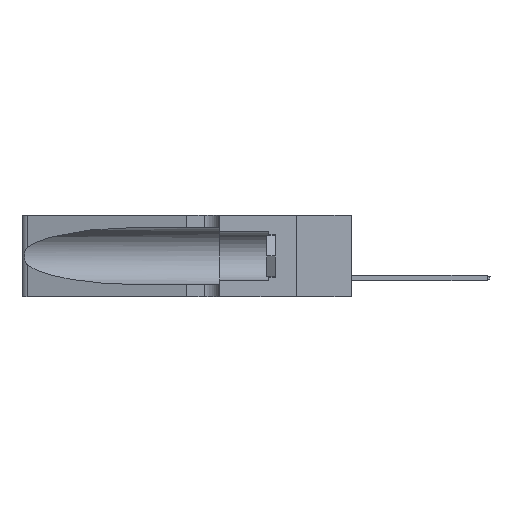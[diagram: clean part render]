
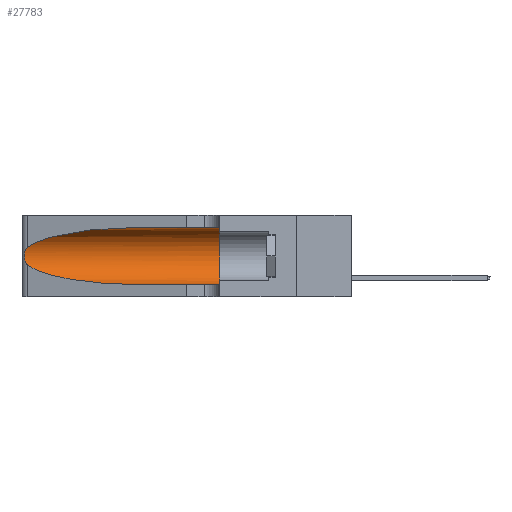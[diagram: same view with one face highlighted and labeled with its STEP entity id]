
A CAD part, left-side view. The second image highlights one B-rep face of the part: STEP entity #27783.
In plain terms, the highlighted cylindrical face has radius 3.308 mm (diameter 6.617 mm), a partial arc.
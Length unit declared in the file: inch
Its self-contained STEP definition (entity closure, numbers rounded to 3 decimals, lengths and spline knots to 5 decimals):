
#856 = DIRECTION ( 'NONE',  ( 0., 0., 1. ) ) ;
#1046 = ORIENTED_EDGE ( 'NONE', *, *, #34919, .F. ) ;
#1336 = CARTESIAN_POINT ( 'NONE',  ( 0.1305, 1.61858, 0.185 ) ) ;
#1360 = CARTESIAN_POINT ( 'NONE',  ( 0.25487, 1.22718, 0.14631 ) ) ;
#1469 = VECTOR ( 'NONE', #13040, 39.37008 ) ;
#3757 = EDGE_CURVE ( 'NONE', #30248, #12861, #10964, .T. ) ;
#3941 = CARTESIAN_POINT ( 'NONE',  ( 0.26017, 1.23833, 0.17102 ) ) ;
#5793 = VERTEX_POINT ( 'NONE', #15947 ) ;
#5950 = VERTEX_POINT ( 'NONE', #10059 ) ;
#6011 = AXIS2_PLACEMENT_3D ( 'NONE', #1336, #27220, #30047 ) ;
#6213 = CYLINDRICAL_SURFACE ( 'NONE', #6011, 0.13025 ) ;
#6783 = VECTOR ( 'NONE', #34614, 39.37008 ) ;
#7017 = EDGE_CURVE ( 'NONE', #27018, #30248, #33963, .T. ) ;
#7101 =( BOUNDED_CURVE ( )  B_SPLINE_CURVE ( 3, ( #36744, #25784, #34082, #22679 ),
 .UNSPECIFIED., .F., .T. ) 
 B_SPLINE_CURVE_WITH_KNOTS ( ( 4, 4 ),
 ( 1.5708, 2.84003 ),
 .UNSPECIFIED. ) 
 CURVE ( )  GEOMETRIC_REPRESENTATION_ITEM ( )  RATIONAL_B_SPLINE_CURVE ( ( 1., 0.87, 0.87, 1. ) ) 
 REPRESENTATION_ITEM ( '' )  );
#9037 = CARTESIAN_POINT ( 'NONE',  ( 0.1305, 0.72297, 0.05475 ) ) ;
#9073 = ORIENTED_EDGE ( 'NONE', *, *, #31526, .T. ) ;
#9606 = CARTESIAN_POINT ( 'NONE',  ( 0.2373, 1.15595, 0.08982 ) ) ;
#9808 = CARTESIAN_POINT ( 'NONE',  ( 0.25787, 1.23484, 0.2124 ) ) ;
#9934 = CARTESIAN_POINT ( 'NONE',  ( 0.25639, 1.23186, 0.15144 ) ) ;
#10059 = CARTESIAN_POINT ( 'NONE',  ( 0.1305, 0.35, 0.31525 ) ) ;
#10964 =( BOUNDED_CURVE ( )  B_SPLINE_CURVE ( 3, ( #29357, #9606, #29480, #21447 ),
 .UNSPECIFIED., .F., .T. ) 
 B_SPLINE_CURVE_WITH_KNOTS ( ( 4, 4 ),
 ( 3.44316, 4.71239 ),
 .UNSPECIFIED. ) 
 CURVE ( )  GEOMETRIC_REPRESENTATION_ITEM ( )  RATIONAL_B_SPLINE_CURVE ( ( 1., 0.87, 0.87, 1. ) ) 
 REPRESENTATION_ITEM ( '' )  );
#11138 = CIRCLE ( 'NONE', #26426, 0.13025 ) ;
#12664 = CARTESIAN_POINT ( 'NONE',  ( 0.25856, 1.23593, 0.16098 ) ) ;
#12861 = VERTEX_POINT ( 'NONE', #9037 ) ;
#13040 = DIRECTION ( 'NONE',  ( 0., -1., 0. ) ) ;
#14253 = CARTESIAN_POINT ( 'NONE',  ( 0.1305, 1.61858, 0.31525 ) ) ;
#15199 = ORIENTED_EDGE ( 'NONE', *, *, #33114, .T. ) ;
#15202 = LINE ( 'NONE', #14253, #6783 ) ;
#15794 = CARTESIAN_POINT ( 'NONE',  ( 0.25487, 1.22718, 0.22369 ) ) ;
#15947 = CARTESIAN_POINT ( 'NONE',  ( 0.1305, 0.72297, 0.31525 ) ) ;
#16217 = EDGE_LOOP ( 'NONE', ( #15199, #35215, #21440, #9073, #18033, #1046 ) ) ;
#18033 = ORIENTED_EDGE ( 'NONE', *, *, #35921, .F. ) ;
#18328 = CARTESIAN_POINT ( 'NONE',  ( 0.25487, 1.22718, 0.14631 ) ) ;
#18377 = CARTESIAN_POINT ( 'NONE',  ( 0.25555, 1.22993, 0.14849 ) ) ;
#18629 = CARTESIAN_POINT ( 'NONE',  ( 0.26075, 1.23896, 0.178 ) ) ;
#20745 = CARTESIAN_POINT ( 'NONE',  ( 0.1305, 0.35, 0.05475 ) ) ;
#21440 = ORIENTED_EDGE ( 'NONE', *, *, #3757, .T. ) ;
#21447 = CARTESIAN_POINT ( 'NONE',  ( 0.1305, 0.72297, 0.05475 ) ) ;
#22679 = CARTESIAN_POINT ( 'NONE',  ( 0.25487, 1.22718, 0.22369 ) ) ;
#24407 = CARTESIAN_POINT ( 'NONE',  ( 0.26018, 1.23835, 0.19895 ) ) ;
#24681 = CARTESIAN_POINT ( 'NONE',  ( 0.1305, 0.35, 0.185 ) ) ;
#24854 = VERTEX_POINT ( 'NONE', #20745 ) ;
#25784 = CARTESIAN_POINT ( 'NONE',  ( 0.18966, 0.96281, 0.31525 ) ) ;
#26426 = AXIS2_PLACEMENT_3D ( 'NONE', #24681, #26498, #856 ) ;
#26498 = DIRECTION ( 'NONE',  ( 0., 1., 0. ) ) ;
#26850 = LINE ( 'NONE', #32785, #1469 ) ;
#27018 = VERTEX_POINT ( 'NONE', #33563 ) ;
#27220 = DIRECTION ( 'NONE',  ( 0., -1., 0. ) ) ;
#27240 = CARTESIAN_POINT ( 'NONE',  ( 0.25639, 1.23184, 0.21858 ) ) ;
#27783 = ADVANCED_FACE ( 'NONE', ( #28398 ), #6213, .F. ) ;
#28398 = FACE_OUTER_BOUND ( 'NONE', #16217, .T. ) ;
#29357 = CARTESIAN_POINT ( 'NONE',  ( 0.25487, 1.22718, 0.14631 ) ) ;
#29480 = CARTESIAN_POINT ( 'NONE',  ( 0.18966, 0.96281, 0.05475 ) ) ;
#29689 = CARTESIAN_POINT ( 'NONE',  ( 0.25854, 1.2359, 0.20912 ) ) ;
#30047 = DIRECTION ( 'NONE',  ( 0., 0., -1. ) ) ;
#30248 = VERTEX_POINT ( 'NONE', #18328 ) ;
#31526 = EDGE_CURVE ( 'NONE', #12861, #24854, #26850, .T. ) ;
#32543 = CARTESIAN_POINT ( 'NONE',  ( 0.25789, 1.23486, 0.15765 ) ) ;
#32785 = CARTESIAN_POINT ( 'NONE',  ( 0.1305, 1.61858, 0.05475 ) ) ;
#33114 = EDGE_CURVE ( 'NONE', #5793, #27018, #7101, .T. ) ;
#33563 = CARTESIAN_POINT ( 'NONE',  ( 0.25487, 1.22718, 0.22369 ) ) ;
#33963 = B_SPLINE_CURVE_WITH_KNOTS ( 'NONE', 3,
 ( #15794, #35696, #27240, #9808, #29689, #24407, #35824, #18629, #3941, #12664, #32543, #9934, #18377, #1360 ),
 .UNSPECIFIED., .F., .F.,
 ( 4, 2, 2, 2, 2, 2, 4 ),
 ( 0., 0.00027, 0.00053, 0.00107, 0.0016, 0.00187, 0.00214 ),
 .UNSPECIFIED. ) ;
#34082 = CARTESIAN_POINT ( 'NONE',  ( 0.2373, 1.15595, 0.28018 ) ) ;
#34614 = DIRECTION ( 'NONE',  ( 0., -1., 0. ) ) ;
#34919 = EDGE_CURVE ( 'NONE', #5793, #5950, #15202, .T. ) ;
#35215 = ORIENTED_EDGE ( 'NONE', *, *, #7017, .T. ) ;
#35696 = CARTESIAN_POINT ( 'NONE',  ( 0.25555, 1.22994, 0.2215 ) ) ;
#35824 = CARTESIAN_POINT ( 'NONE',  ( 0.26075, 1.23896, 0.19203 ) ) ;
#35921 = EDGE_CURVE ( 'NONE', #5950, #24854, #11138, .T. ) ;
#36744 = CARTESIAN_POINT ( 'NONE',  ( 0.1305, 0.72297, 0.31525 ) ) ;
